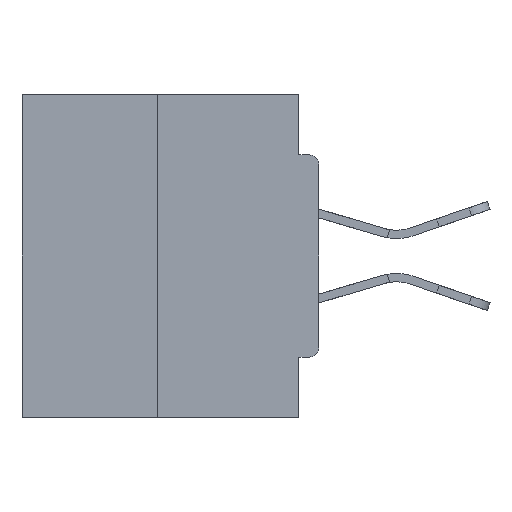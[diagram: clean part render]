
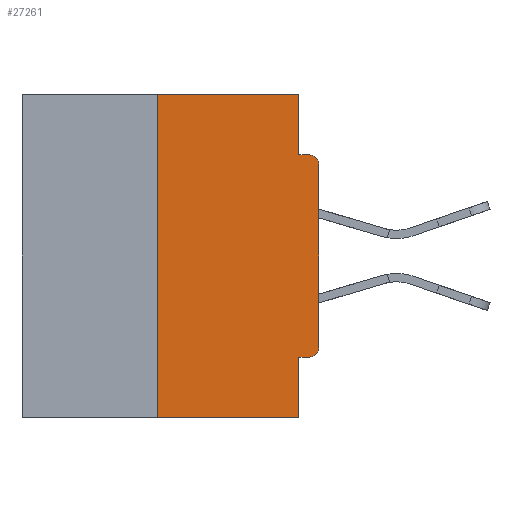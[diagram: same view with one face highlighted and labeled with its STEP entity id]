
A CAD part, left-side view. The second image highlights one B-rep face of the part: STEP entity #27261.
In plain terms, the highlighted planar face has unit normal (-1, 0, 0).
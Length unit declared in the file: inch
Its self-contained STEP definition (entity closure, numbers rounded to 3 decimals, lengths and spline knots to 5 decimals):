
#66 = LINE ( 'NONE', #27712, #33312 ) ;
#74 = DIRECTION ( 'NONE',  ( 0., 0., -1. ) ) ;
#592 = DIRECTION ( 'NONE',  ( 0., -1., 0. ) ) ;
#795 = LINE ( 'NONE', #28783, #31887 ) ;
#1105 = EDGE_CURVE ( 'NONE', #34471, #1715, #795, .T. ) ;
#1715 = VERTEX_POINT ( 'NONE', #9773 ) ;
#2035 = ORIENTED_EDGE ( 'NONE', *, *, #1105, .F. ) ;
#2328 = EDGE_LOOP ( 'NONE', ( #16761, #3167, #22607, #14597, #11487, #33893, #38335, #33031, #2035, #6582 ) ) ;
#2455 = AXIS2_PLACEMENT_3D ( 'NONE', #18358, #32346, #41921 ) ;
#3167 = ORIENTED_EDGE ( 'NONE', *, *, #35551, .F. ) ;
#4946 = VERTEX_POINT ( 'NONE', #27029 ) ;
#6582 = ORIENTED_EDGE ( 'NONE', *, *, #25408, .F. ) ;
#6608 = DIRECTION ( 'NONE',  ( 0., 0., -1. ) ) ;
#6971 = VECTOR ( 'NONE', #21987, 39.37008 ) ;
#7499 = LINE ( 'NONE', #8673, #6971 ) ;
#7902 = LINE ( 'NONE', #41134, #32049 ) ;
#8601 = VERTEX_POINT ( 'NONE', #24525 ) ;
#8673 = CARTESIAN_POINT ( 'NONE',  ( 0., 0.25, 0. ) ) ;
#9216 = LINE ( 'NONE', #31740, #42444 ) ;
#9773 = CARTESIAN_POINT ( 'NONE',  ( 0., 0.015, -0.0935 ) ) ;
#10401 = DIRECTION ( 'NONE',  ( 0., 0., 1. ) ) ;
#11487 = ORIENTED_EDGE ( 'NONE', *, *, #27230, .F. ) ;
#13317 = EDGE_CURVE ( 'NONE', #13781, #4946, #17624, .T. ) ;
#13781 = VERTEX_POINT ( 'NONE', #16397 ) ;
#14170 = CARTESIAN_POINT ( 'NONE',  ( 0., 0.46, 0. ) ) ;
#14597 = ORIENTED_EDGE ( 'NONE', *, *, #19557, .F. ) ;
#16397 = CARTESIAN_POINT ( 'NONE',  ( 0., 0.015, -0.4065 ) ) ;
#16761 = ORIENTED_EDGE ( 'NONE', *, *, #32300, .F. ) ;
#17624 = CIRCLE ( 'NONE', #36472, 0.015 ) ;
#17742 = CARTESIAN_POINT ( 'NONE',  ( 0., 0.25, 0. ) ) ;
#18358 = CARTESIAN_POINT ( 'NONE',  ( 0., 0.46, 0. ) ) ;
#18654 = VERTEX_POINT ( 'NONE', #36434 ) ;
#19489 = CIRCLE ( 'NONE', #20117, 0.015 ) ;
#19557 = EDGE_CURVE ( 'NONE', #8601, #31775, #43518, .T. ) ;
#20117 = AXIS2_PLACEMENT_3D ( 'NONE', #42772, #28837, #25787 ) ;
#21638 = VERTEX_POINT ( 'NONE', #17742 ) ;
#21987 = DIRECTION ( 'NONE',  ( 0., 0., 1. ) ) ;
#22607 = ORIENTED_EDGE ( 'NONE', *, *, #30954, .T. ) ;
#24307 = EDGE_CURVE ( 'NONE', #39156, #1715, #19489, .T. ) ;
#24525 = CARTESIAN_POINT ( 'NONE',  ( 0., 0.031, -0.4065 ) ) ;
#24676 = CARTESIAN_POINT ( 'NONE',  ( 0., 0., -0.1085 ) ) ;
#25408 = EDGE_CURVE ( 'NONE', #27656, #34471, #7902, .T. ) ;
#25787 = DIRECTION ( 'NONE',  ( 0., 0., -1. ) ) ;
#27029 = CARTESIAN_POINT ( 'NONE',  ( 0., 0., -0.3915 ) ) ;
#27230 = EDGE_CURVE ( 'NONE', #13781, #8601, #9216, .T. ) ;
#27261 = ADVANCED_FACE ( 'NONE', ( #40642 ), #42086, .F. ) ;
#27656 = VERTEX_POINT ( 'NONE', #34299 ) ;
#27712 = CARTESIAN_POINT ( 'NONE',  ( 0., 0.46, -0.5 ) ) ;
#28783 = CARTESIAN_POINT ( 'NONE',  ( 0., 0., -0.0935 ) ) ;
#28837 = DIRECTION ( 'NONE',  ( -1., 0., 0. ) ) ;
#29826 = EDGE_CURVE ( 'NONE', #4946, #39156, #34006, .T. ) ;
#30954 = EDGE_CURVE ( 'NONE', #18654, #31775, #66, .T. ) ;
#31740 = CARTESIAN_POINT ( 'NONE',  ( 0., 0., -0.4065 ) ) ;
#31775 = VERTEX_POINT ( 'NONE', #42634 ) ;
#31887 = VECTOR ( 'NONE', #35822, 39.37008 ) ;
#32049 = VECTOR ( 'NONE', #74, 39.37008 ) ;
#32300 = EDGE_CURVE ( 'NONE', #21638, #27656, #37530, .T. ) ;
#32346 = DIRECTION ( 'NONE',  ( 1., 0., 0. ) ) ;
#33031 = ORIENTED_EDGE ( 'NONE', *, *, #24307, .T. ) ;
#33312 = VECTOR ( 'NONE', #592, 39.37008 ) ;
#33893 = ORIENTED_EDGE ( 'NONE', *, *, #13317, .T. ) ;
#34006 = LINE ( 'NONE', #36183, #44178 ) ;
#34299 = CARTESIAN_POINT ( 'NONE',  ( 0., 0.031, 0. ) ) ;
#34471 = VERTEX_POINT ( 'NONE', #34956 ) ;
#34956 = CARTESIAN_POINT ( 'NONE',  ( 0., 0.031, -0.0935 ) ) ;
#35551 = EDGE_CURVE ( 'NONE', #18654, #21638, #7499, .T. ) ;
#35822 = DIRECTION ( 'NONE',  ( 0., -1., 0. ) ) ;
#36183 = CARTESIAN_POINT ( 'NONE',  ( 0., 0., 0. ) ) ;
#36434 = CARTESIAN_POINT ( 'NONE',  ( 0., 0.25, -0.5 ) ) ;
#36472 = AXIS2_PLACEMENT_3D ( 'NONE', #37466, #43897, #6608 ) ;
#37466 = CARTESIAN_POINT ( 'NONE',  ( 0., 0.015, -0.3915 ) ) ;
#37484 = DIRECTION ( 'NONE',  ( 0., 0., -1. ) ) ;
#37530 = LINE ( 'NONE', #14170, #38581 ) ;
#38335 = ORIENTED_EDGE ( 'NONE', *, *, #29826, .T. ) ;
#38581 = VECTOR ( 'NONE', #41771, 39.37008 ) ;
#38911 = DIRECTION ( 'NONE',  ( 0., 1., 0. ) ) ;
#39156 = VERTEX_POINT ( 'NONE', #24676 ) ;
#39809 = VECTOR ( 'NONE', #37484, 39.37008 ) ;
#40336 = CARTESIAN_POINT ( 'NONE',  ( 0., 0.031, -0.5 ) ) ;
#40642 = FACE_OUTER_BOUND ( 'NONE', #2328, .T. ) ;
#41134 = CARTESIAN_POINT ( 'NONE',  ( 0., 0.031, 0. ) ) ;
#41771 = DIRECTION ( 'NONE',  ( 0., -1., 0. ) ) ;
#41921 = DIRECTION ( 'NONE',  ( 0., 0., -1. ) ) ;
#42086 = PLANE ( 'NONE',  #2455 ) ;
#42444 = VECTOR ( 'NONE', #38911, 39.37008 ) ;
#42634 = CARTESIAN_POINT ( 'NONE',  ( 0., 0.031, -0.5 ) ) ;
#42772 = CARTESIAN_POINT ( 'NONE',  ( 0., 0.015, -0.1085 ) ) ;
#43518 = LINE ( 'NONE', #40336, #39809 ) ;
#43897 = DIRECTION ( 'NONE',  ( -1., 0., 0. ) ) ;
#44178 = VECTOR ( 'NONE', #10401, 39.37008 ) ;
